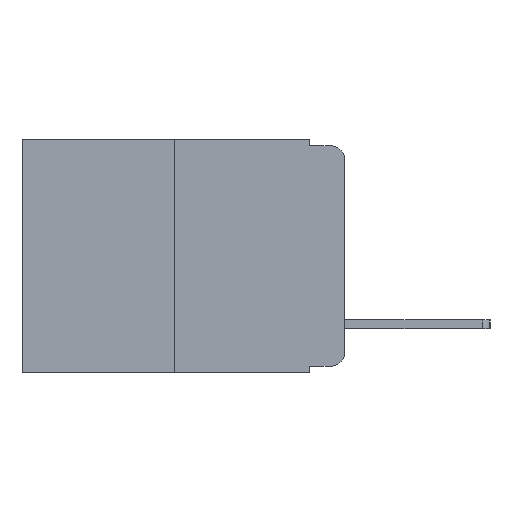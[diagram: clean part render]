
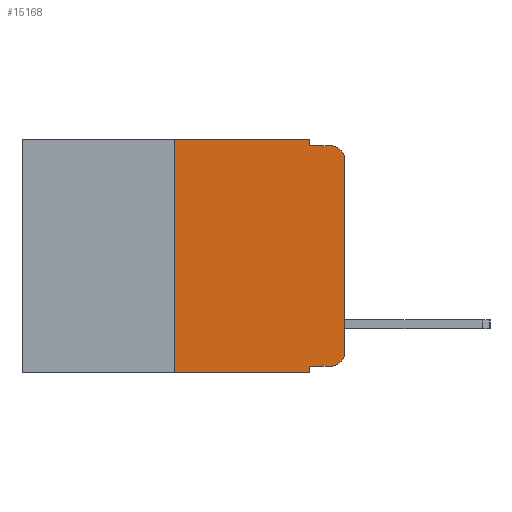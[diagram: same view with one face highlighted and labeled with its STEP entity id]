
A CAD part, left-side view. The second image highlights one B-rep face of the part: STEP entity #15168.
In plain terms, the highlighted planar face has unit normal (-1, 0, 0).
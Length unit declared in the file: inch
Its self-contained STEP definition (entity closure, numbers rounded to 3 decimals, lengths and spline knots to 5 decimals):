
#129 = EDGE_CURVE ( 'NONE', #2720, #6043, #10554, .T. ) ;
#306 = VERTEX_POINT ( 'NONE', #23106 ) ;
#500 = CARTESIAN_POINT ( 'NONE',  ( 0., 0.051, -0.333 ) ) ;
#671 = LINE ( 'NONE', #23798, #4975 ) ;
#919 = VERTEX_POINT ( 'NONE', #9321 ) ;
#975 = VERTEX_POINT ( 'NONE', #500 ) ;
#1227 = CIRCLE ( 'NONE', #24061, 0.02 ) ;
#1451 = VERTEX_POINT ( 'NONE', #12706 ) ;
#1956 = ORIENTED_EDGE ( 'NONE', *, *, #14121, .T. ) ;
#2035 = CARTESIAN_POINT ( 'NONE',  ( 0., 0.051, -0.01 ) ) ;
#2069 = CARTESIAN_POINT ( 'NONE',  ( 0., 0.473, 0. ) ) ;
#2720 = VERTEX_POINT ( 'NONE', #17219 ) ;
#2796 = DIRECTION ( 'NONE',  ( -1., 0., 0. ) ) ;
#2984 = DIRECTION ( 'NONE',  ( 0., -1., 0. ) ) ;
#4218 = DIRECTION ( 'NONE',  ( 0., 0., -1. ) ) ;
#4278 = ORIENTED_EDGE ( 'NONE', *, *, #129, .F. ) ;
#4840 = CARTESIAN_POINT ( 'NONE',  ( 0., 0., 0. ) ) ;
#4924 = DIRECTION ( 'NONE',  ( 0., 0., 1. ) ) ;
#4975 = VECTOR ( 'NONE', #25705, 39.37008 ) ;
#5801 = EDGE_CURVE ( 'NONE', #10214, #919, #671, .T. ) ;
#6043 = VERTEX_POINT ( 'NONE', #16822 ) ;
#6099 = CARTESIAN_POINT ( 'NONE',  ( 0., 0., -0.313 ) ) ;
#6989 = AXIS2_PLACEMENT_3D ( 'NONE', #21834, #10078, #23757 ) ;
#7092 = CARTESIAN_POINT ( 'NONE',  ( 0., 0.473, 0. ) ) ;
#7177 = EDGE_CURVE ( 'NONE', #919, #1451, #24725, .T. ) ;
#8696 = CARTESIAN_POINT ( 'NONE',  ( 0., 0.051, -0.333 ) ) ;
#8849 = LINE ( 'NONE', #8696, #20600 ) ;
#9321 = CARTESIAN_POINT ( 'NONE',  ( 0., 0.051, -0.01 ) ) ;
#10078 = DIRECTION ( 'NONE',  ( -1., 0., 0. ) ) ;
#10214 = VERTEX_POINT ( 'NONE', #14463 ) ;
#10327 = AXIS2_PLACEMENT_3D ( 'NONE', #2069, #16380, #4218 ) ;
#10408 = ORIENTED_EDGE ( 'NONE', *, *, #20705, .T. ) ;
#10554 = LINE ( 'NONE', #14804, #25496 ) ;
#12263 = EDGE_CURVE ( 'NONE', #975, #17139, #8849, .T. ) ;
#12498 = CARTESIAN_POINT ( 'NONE',  ( 0., 0.051, 0. ) ) ;
#12706 = CARTESIAN_POINT ( 'NONE',  ( 0., 0.02, -0.01 ) ) ;
#13449 = VECTOR ( 'NONE', #14511, 39.37008 ) ;
#13970 = VECTOR ( 'NONE', #2984, 39.37008 ) ;
#14121 = EDGE_CURVE ( 'NONE', #17139, #19289, #1227, .T. ) ;
#14463 = CARTESIAN_POINT ( 'NONE',  ( 0., 0.051, 0. ) ) ;
#14511 = DIRECTION ( 'NONE',  ( 0., 0., -1. ) ) ;
#14707 = CARTESIAN_POINT ( 'NONE',  ( 0., 0.473, -0.343 ) ) ;
#14804 = CARTESIAN_POINT ( 'NONE',  ( 0., 0.25, 0. ) ) ;
#15042 = CARTESIAN_POINT ( 'NONE',  ( 0., 0.02, -0.313 ) ) ;
#15168 = ADVANCED_FACE ( 'NONE', ( #22567 ), #22073, .F. ) ;
#15736 = ORIENTED_EDGE ( 'NONE', *, *, #15791, .F. ) ;
#15791 = EDGE_CURVE ( 'NONE', #975, #306, #24355, .T. ) ;
#15886 = EDGE_LOOP ( 'NONE', ( #25614, #25634, #17257, #18445, #24761, #4278, #10408, #15736, #16966, #1956 ) ) ;
#16056 = CARTESIAN_POINT ( 'NONE',  ( 0., 0., -0.03 ) ) ;
#16352 = DIRECTION ( 'NONE',  ( 0., -1., 0. ) ) ;
#16380 = DIRECTION ( 'NONE',  ( 1., 0., 0. ) ) ;
#16664 = DIRECTION ( 'NONE',  ( 0., -1., 0. ) ) ;
#16697 = DIRECTION ( 'NONE',  ( 0., -1., 0. ) ) ;
#16822 = CARTESIAN_POINT ( 'NONE',  ( 0., 0.25, 0. ) ) ;
#16966 = ORIENTED_EDGE ( 'NONE', *, *, #12263, .T. ) ;
#17015 = DIRECTION ( 'NONE',  ( 0., 0., -1. ) ) ;
#17139 = VERTEX_POINT ( 'NONE', #19077 ) ;
#17219 = CARTESIAN_POINT ( 'NONE',  ( 0., 0.25, -0.343 ) ) ;
#17257 = ORIENTED_EDGE ( 'NONE', *, *, #7177, .F. ) ;
#17680 = EDGE_CURVE ( 'NONE', #6043, #10214, #19175, .T. ) ;
#17800 = LINE ( 'NONE', #14707, #22290 ) ;
#18445 = ORIENTED_EDGE ( 'NONE', *, *, #5801, .F. ) ;
#19077 = CARTESIAN_POINT ( 'NONE',  ( 0., 0.02, -0.333 ) ) ;
#19175 = LINE ( 'NONE', #7092, #13970 ) ;
#19289 = VERTEX_POINT ( 'NONE', #6099 ) ;
#19638 = VECTOR ( 'NONE', #16352, 39.37008 ) ;
#20489 = EDGE_CURVE ( 'NONE', #25413, #1451, #22607, .T. ) ;
#20600 = VECTOR ( 'NONE', #16664, 39.37008 ) ;
#20705 = EDGE_CURVE ( 'NONE', #2720, #306, #17800, .T. ) ;
#20832 = DIRECTION ( 'NONE',  ( 0., 0., 1. ) ) ;
#21834 = CARTESIAN_POINT ( 'NONE',  ( 0., 0.02, -0.03 ) ) ;
#22073 = PLANE ( 'NONE',  #10327 ) ;
#22290 = VECTOR ( 'NONE', #16697, 39.37008 ) ;
#22567 = FACE_OUTER_BOUND ( 'NONE', #15886, .T. ) ;
#22607 = CIRCLE ( 'NONE', #6989, 0.02 ) ;
#23106 = CARTESIAN_POINT ( 'NONE',  ( 0., 0.051, -0.343 ) ) ;
#23366 = VECTOR ( 'NONE', #4924, 39.37008 ) ;
#23757 = DIRECTION ( 'NONE',  ( 0., 0., -1. ) ) ;
#23798 = CARTESIAN_POINT ( 'NONE',  ( 0., 0.051, 0. ) ) ;
#24061 = AXIS2_PLACEMENT_3D ( 'NONE', #15042, #2796, #17015 ) ;
#24331 = EDGE_CURVE ( 'NONE', #19289, #25413, #24564, .T. ) ;
#24355 = LINE ( 'NONE', #12498, #13449 ) ;
#24564 = LINE ( 'NONE', #4840, #23366 ) ;
#24725 = LINE ( 'NONE', #2035, #19638 ) ;
#24761 = ORIENTED_EDGE ( 'NONE', *, *, #17680, .F. ) ;
#25413 = VERTEX_POINT ( 'NONE', #16056 ) ;
#25496 = VECTOR ( 'NONE', #20832, 39.37008 ) ;
#25614 = ORIENTED_EDGE ( 'NONE', *, *, #24331, .T. ) ;
#25634 = ORIENTED_EDGE ( 'NONE', *, *, #20489, .T. ) ;
#25705 = DIRECTION ( 'NONE',  ( 0., 0., -1. ) ) ;
